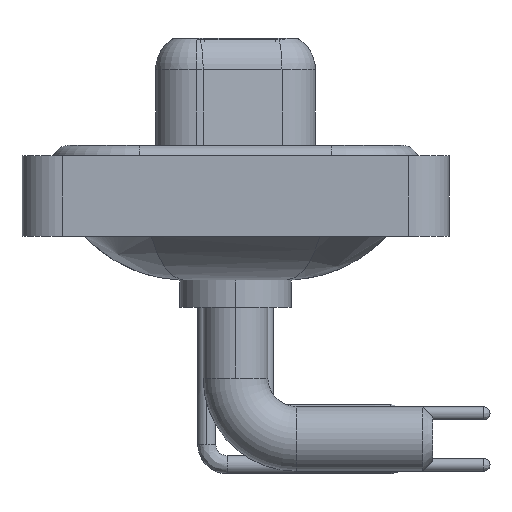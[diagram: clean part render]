
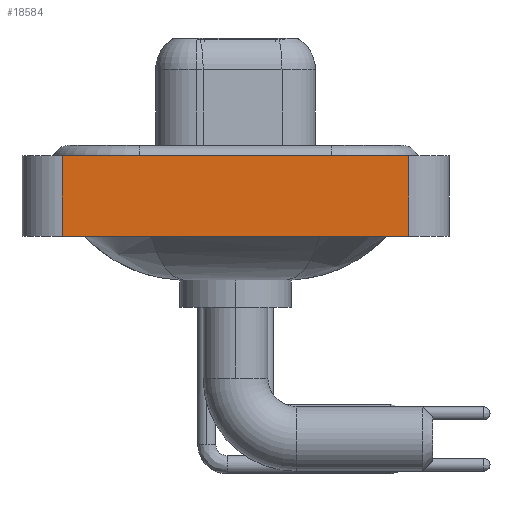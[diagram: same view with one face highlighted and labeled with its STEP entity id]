
A CAD part, left-side view. The second image highlights one B-rep face of the part: STEP entity #18584.
In plain terms, the highlighted planar face has unit normal (-1, 0, 0).
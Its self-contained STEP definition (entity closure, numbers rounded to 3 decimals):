
#465 = LINE ( 'NONE', #17507, #17620 ) ;
#1156 = CARTESIAN_POINT ( 'NONE',  ( -7.3, -8.55, 0.4 ) ) ;
#2962 = DIRECTION ( 'NONE',  ( 0., 0., 1. ) ) ;
#4907 = CARTESIAN_POINT ( 'NONE',  ( -7.3, -8.55, -3.6 ) ) ;
#5844 = ORIENTED_EDGE ( 'NONE', *, *, #16510, .T. ) ;
#6088 = LINE ( 'NONE', #12671, #20472 ) ;
#6439 = VECTOR ( 'NONE', #9409, 1000. ) ;
#6495 = CARTESIAN_POINT ( 'NONE',  ( -7.3, -8.55, 0.4 ) ) ;
#6560 = CARTESIAN_POINT ( 'NONE',  ( -7.3, 8.55, -3.6 ) ) ;
#6617 = DIRECTION ( 'NONE',  ( 0., 0., 1. ) ) ;
#6973 = CARTESIAN_POINT ( 'NONE',  ( -7.3, 8.55, -3.6 ) ) ;
#7696 = EDGE_CURVE ( 'NONE', #12058, #12688, #6088, .T. ) ;
#7945 = ORIENTED_EDGE ( 'NONE', *, *, #7696, .T. ) ;
#9409 = DIRECTION ( 'NONE',  ( 0., -1., 0. ) ) ;
#9605 = FACE_OUTER_BOUND ( 'NONE', #12963, .T. ) ;
#10751 = LINE ( 'NONE', #1156, #6439 ) ;
#11930 = VERTEX_POINT ( 'NONE', #12047 ) ;
#12047 = CARTESIAN_POINT ( 'NONE',  ( -7.3, 8.55, 0.4 ) ) ;
#12058 = VERTEX_POINT ( 'NONE', #4907 ) ;
#12539 = ORIENTED_EDGE ( 'NONE', *, *, #18521, .F. ) ;
#12671 = CARTESIAN_POINT ( 'NONE',  ( -7.3, -8.55, -3.6 ) ) ;
#12688 = VERTEX_POINT ( 'NONE', #6495 ) ;
#12963 = EDGE_LOOP ( 'NONE', ( #7945, #12539, #20419, #5844 ) ) ;
#13011 = CARTESIAN_POINT ( 'NONE',  ( -7.3, -8.55, -3.6 ) ) ;
#14345 = AXIS2_PLACEMENT_3D ( 'NONE', #13011, #17763, #6617 ) ;
#14755 = EDGE_CURVE ( 'NONE', #16467, #11930, #17933, .T. ) ;
#15518 = VECTOR ( 'NONE', #16259, 1000. ) ;
#15905 = PLANE ( 'NONE',  #14345 ) ;
#16259 = DIRECTION ( 'NONE',  ( 0., 0., 1. ) ) ;
#16467 = VERTEX_POINT ( 'NONE', #6560 ) ;
#16510 = EDGE_CURVE ( 'NONE', #16467, #12058, #465, .T. ) ;
#17507 = CARTESIAN_POINT ( 'NONE',  ( -7.3, -8.55, -3.6 ) ) ;
#17620 = VECTOR ( 'NONE', #18112, 1000. ) ;
#17763 = DIRECTION ( 'NONE',  ( -1., 0., 0. ) ) ;
#17933 = LINE ( 'NONE', #6973, #15518 ) ;
#18112 = DIRECTION ( 'NONE',  ( 0., -1., 0. ) ) ;
#18521 = EDGE_CURVE ( 'NONE', #11930, #12688, #10751, .T. ) ;
#18584 = ADVANCED_FACE ( 'NONE', ( #9605 ), #15905, .T. ) ;
#20419 = ORIENTED_EDGE ( 'NONE', *, *, #14755, .F. ) ;
#20472 = VECTOR ( 'NONE', #2962, 1000. ) ;
